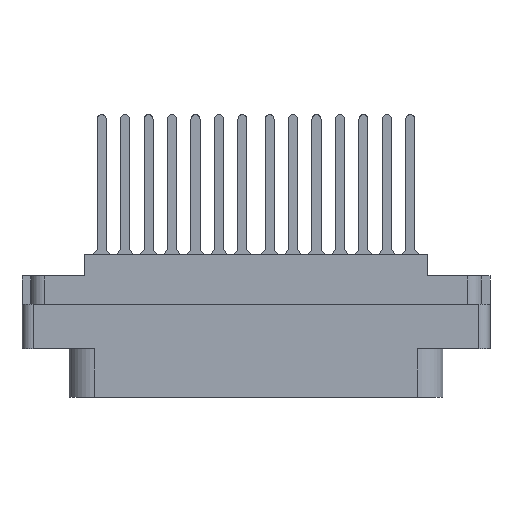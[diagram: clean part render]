
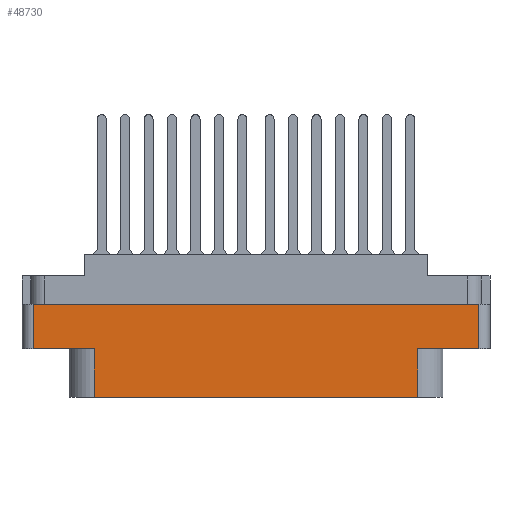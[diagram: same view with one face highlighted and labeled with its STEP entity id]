
A CAD part, front view. The second image highlights one B-rep face of the part: STEP entity #48730.
In plain terms, the highlighted planar face has unit normal (0, -1, 0).
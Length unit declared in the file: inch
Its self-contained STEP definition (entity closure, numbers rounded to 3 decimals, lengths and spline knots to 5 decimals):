
#567 = LINE ( 'NONE', #31254, #31067 ) ;
#1831 = VERTEX_POINT ( 'NONE', #35962 ) ;
#1894 = EDGE_CURVE ( 'NONE', #17253, #1831, #26887, .T. ) ;
#2818 = VECTOR ( 'NONE', #12646, 39.37008 ) ;
#3251 = DIRECTION ( 'NONE',  ( -1., 0., 0. ) ) ;
#5580 = VECTOR ( 'NONE', #27629, 39.37008 ) ;
#6314 = CARTESIAN_POINT ( 'NONE',  ( 0.895, -0.438, -0.52 ) ) ;
#7317 = ORIENTED_EDGE ( 'NONE', *, *, #15261, .F. ) ;
#7944 = CARTESIAN_POINT ( 'NONE',  ( 0.895, -0.438, -0.52 ) ) ;
#8979 = DIRECTION ( 'NONE',  ( -1., 0., 0. ) ) ;
#9247 = LINE ( 'NONE', #7944, #38510 ) ;
#9290 = EDGE_CURVE ( 'NONE', #28195, #21206, #9247, .T. ) ;
#9292 = EDGE_CURVE ( 'NONE', #19817, #19765, #15201, .T. ) ;
#9399 = VECTOR ( 'NONE', #3251, 39.37008 ) ;
#9619 = CARTESIAN_POINT ( 'NONE',  ( -0.895, -0.438, -0.52 ) ) ;
#11413 = EDGE_CURVE ( 'NONE', #17253, #19765, #19506, .T. ) ;
#12047 = ORIENTED_EDGE ( 'NONE', *, *, #22742, .T. ) ;
#12263 = DIRECTION ( 'NONE',  ( 0., 0., 1. ) ) ;
#12646 = DIRECTION ( 'NONE',  ( 1., 0., 0. ) ) ;
#13200 = PLANE ( 'NONE',  #42111 ) ;
#13604 = CARTESIAN_POINT ( 'NONE',  ( 0., -0.438, -0.274 ) ) ;
#14240 = CARTESIAN_POINT ( 'NONE',  ( -0.895, -0.438, -0.789 ) ) ;
#14316 = CARTESIAN_POINT ( 'NONE',  ( -1.2335, -0.438, -0.52 ) ) ;
#14612 = CARTESIAN_POINT ( 'NONE',  ( 0.895, -0.438, -0.789 ) ) ;
#15201 = LINE ( 'NONE', #30974, #5580 ) ;
#15261 = EDGE_CURVE ( 'NONE', #19817, #25862, #17082, .T. ) ;
#17082 = LINE ( 'NONE', #13604, #43388 ) ;
#17253 = VERTEX_POINT ( 'NONE', #9619 ) ;
#17305 = VECTOR ( 'NONE', #40945, 39.37008 ) ;
#17440 = DIRECTION ( 'NONE',  ( 1., 0., 0. ) ) ;
#17893 = ORIENTED_EDGE ( 'NONE', *, *, #48122, .F. ) ;
#19506 = LINE ( 'NONE', #37883, #9399 ) ;
#19765 = VERTEX_POINT ( 'NONE', #14316 ) ;
#19817 = VERTEX_POINT ( 'NONE', #49011 ) ;
#20054 = DIRECTION ( 'NONE',  ( 0., 0., 1. ) ) ;
#20821 = DIRECTION ( 'NONE',  ( 0., 0., -1. ) ) ;
#21206 = VERTEX_POINT ( 'NONE', #6314 ) ;
#22742 = EDGE_CURVE ( 'NONE', #34409, #25862, #567, .T. ) ;
#23962 = CARTESIAN_POINT ( 'NONE',  ( 0., -0.438, -0.52 ) ) ;
#25024 = EDGE_LOOP ( 'NONE', ( #7317, #29538, #35590, #36211, #27201, #39423, #17893, #12047 ) ) ;
#25862 = VERTEX_POINT ( 'NONE', #39506 ) ;
#26887 = LINE ( 'NONE', #14240, #17305 ) ;
#27201 = ORIENTED_EDGE ( 'NONE', *, *, #48058, .T. ) ;
#27629 = DIRECTION ( 'NONE',  ( 0., 0., -1. ) ) ;
#28195 = VERTEX_POINT ( 'NONE', #14612 ) ;
#29538 = ORIENTED_EDGE ( 'NONE', *, *, #9292, .T. ) ;
#30974 = CARTESIAN_POINT ( 'NONE',  ( -1.2335, -0.438, -0.789 ) ) ;
#31067 = VECTOR ( 'NONE', #12263, 39.37008 ) ;
#31254 = CARTESIAN_POINT ( 'NONE',  ( 1.2335, -0.438, -0.789 ) ) ;
#34409 = VERTEX_POINT ( 'NONE', #43875 ) ;
#34990 = CARTESIAN_POINT ( 'NONE',  ( -1.2955, -0.438, -0.789 ) ) ;
#35590 = ORIENTED_EDGE ( 'NONE', *, *, #11413, .F. ) ;
#35962 = CARTESIAN_POINT ( 'NONE',  ( -0.895, -0.438, -0.789 ) ) ;
#36211 = ORIENTED_EDGE ( 'NONE', *, *, #1894, .T. ) ;
#36962 = LINE ( 'NONE', #23962, #39923 ) ;
#37525 = LINE ( 'NONE', #34990, #2818 ) ;
#37883 = CARTESIAN_POINT ( 'NONE',  ( 0., -0.438, -0.52 ) ) ;
#38120 = FACE_OUTER_BOUND ( 'NONE', #25024, .T. ) ;
#38510 = VECTOR ( 'NONE', #20054, 39.37008 ) ;
#39423 = ORIENTED_EDGE ( 'NONE', *, *, #9290, .T. ) ;
#39506 = CARTESIAN_POINT ( 'NONE',  ( 1.2335, -0.438, -0.274 ) ) ;
#39896 = CARTESIAN_POINT ( 'NONE',  ( -1.2955, -0.438, -0.789 ) ) ;
#39923 = VECTOR ( 'NONE', #8979, 39.37008 ) ;
#40945 = DIRECTION ( 'NONE',  ( 0., 0., -1. ) ) ;
#42111 = AXIS2_PLACEMENT_3D ( 'NONE', #39896, #43733, #20821 ) ;
#43388 = VECTOR ( 'NONE', #17440, 39.37008 ) ;
#43733 = DIRECTION ( 'NONE',  ( 0., -1., 0. ) ) ;
#43875 = CARTESIAN_POINT ( 'NONE',  ( 1.2335, -0.438, -0.52 ) ) ;
#48058 = EDGE_CURVE ( 'NONE', #1831, #28195, #37525, .T. ) ;
#48122 = EDGE_CURVE ( 'NONE', #34409, #21206, #36962, .T. ) ;
#48730 = ADVANCED_FACE ( 'NONE', ( #38120 ), #13200, .T. ) ;
#49011 = CARTESIAN_POINT ( 'NONE',  ( -1.2335, -0.438, -0.274 ) ) ;
